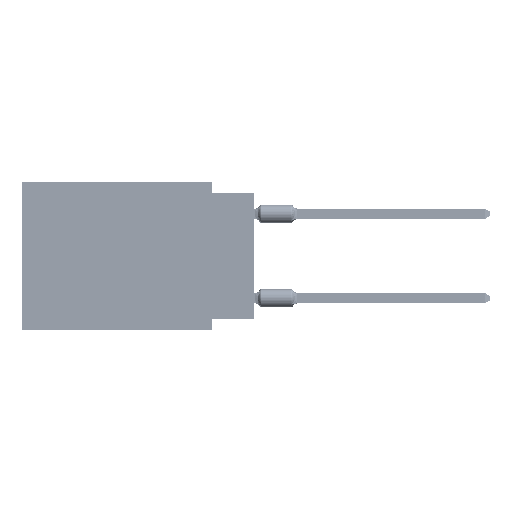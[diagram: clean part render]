
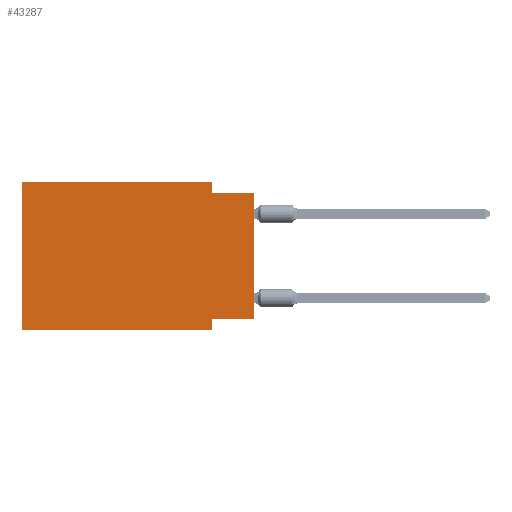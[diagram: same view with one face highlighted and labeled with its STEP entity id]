
A CAD part, left-side view. The second image highlights one B-rep face of the part: STEP entity #43287.
In plain terms, the highlighted planar face has unit normal (-1, 0, 0).
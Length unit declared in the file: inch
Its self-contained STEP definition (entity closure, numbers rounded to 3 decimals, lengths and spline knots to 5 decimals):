
#4055 = VECTOR ( 'NONE', #71321, 39.37008 ) ;
#4350 = VERTEX_POINT ( 'NONE', #39939 ) ;
#8627 = LINE ( 'NONE', #108207, #74319 ) ;
#8752 = VERTEX_POINT ( 'NONE', #32799 ) ;
#10209 = CARTESIAN_POINT ( 'NONE',  ( 0., 0., -0.025 ) ) ;
#11160 = DIRECTION ( 'NONE',  ( 0., 0., 1. ) ) ;
#11512 = CARTESIAN_POINT ( 'NONE',  ( 0., 0., -0.325 ) ) ;
#12114 = CARTESIAN_POINT ( 'NONE',  ( 0., 0.55, -0.35 ) ) ;
#12260 = ORIENTED_EDGE ( 'NONE', *, *, #32055, .T. ) ;
#14042 = VERTEX_POINT ( 'NONE', #77838 ) ;
#15272 = VECTOR ( 'NONE', #106214, 39.37008 ) ;
#15447 = EDGE_CURVE ( 'NONE', #56225, #14042, #8627, .T. ) ;
#16925 = DIRECTION ( 'NONE',  ( 0., 0., -1. ) ) ;
#19380 = ORIENTED_EDGE ( 'NONE', *, *, #62951, .F. ) ;
#21903 = VERTEX_POINT ( 'NONE', #11512 ) ;
#22581 = ORIENTED_EDGE ( 'NONE', *, *, #30645, .F. ) ;
#22696 = LINE ( 'NONE', #89085, #15272 ) ;
#24093 = CARTESIAN_POINT ( 'NONE',  ( 0., 0.1, -0.325 ) ) ;
#24596 = VECTOR ( 'NONE', #11160, 39.37008 ) ;
#25151 = CARTESIAN_POINT ( 'NONE',  ( 0., 0.55, 0. ) ) ;
#25230 = EDGE_CURVE ( 'NONE', #21903, #105555, #95223, .T. ) ;
#25435 = CARTESIAN_POINT ( 'NONE',  ( 0., 0., -0.325 ) ) ;
#25860 = DIRECTION ( 'NONE',  ( 0., -1., 0. ) ) ;
#29530 = CARTESIAN_POINT ( 'NONE',  ( 0., 0.55, 0. ) ) ;
#29986 = ORIENTED_EDGE ( 'NONE', *, *, #70982, .F. ) ;
#30645 = EDGE_CURVE ( 'NONE', #21903, #56225, #42617, .T. ) ;
#32055 = EDGE_CURVE ( 'NONE', #38311, #14042, #88986, .T. ) ;
#32799 = CARTESIAN_POINT ( 'NONE',  ( 0., 0.55, 0. ) ) ;
#32809 = AXIS2_PLACEMENT_3D ( 'NONE', #25151, #92608, #77106 ) ;
#34177 = LINE ( 'NONE', #67895, #62519 ) ;
#37190 = VECTOR ( 'NONE', #96983, 39.37008 ) ;
#38311 = VERTEX_POINT ( 'NONE', #40874 ) ;
#39939 = CARTESIAN_POINT ( 'NONE',  ( 0., 0.1, -0.025 ) ) ;
#40874 = CARTESIAN_POINT ( 'NONE',  ( 0., 0.55, -0.35 ) ) ;
#42617 = LINE ( 'NONE', #25435, #72996 ) ;
#43287 = ADVANCED_FACE ( 'NONE', ( #102017 ), #100930, .F. ) ;
#43338 = EDGE_LOOP ( 'NONE', ( #56687, #19380, #85348, #29986, #90044, #12260, #63796, #22581 ) ) ;
#49837 = EDGE_CURVE ( 'NONE', #90255, #4350, #76809, .T. ) ;
#56225 = VERTEX_POINT ( 'NONE', #24093 ) ;
#56687 = ORIENTED_EDGE ( 'NONE', *, *, #25230, .T. ) ;
#56701 = EDGE_CURVE ( 'NONE', #38311, #8752, #22696, .T. ) ;
#59151 = DIRECTION ( 'NONE',  ( 0., 0., -1. ) ) ;
#62519 = VECTOR ( 'NONE', #25860, 39.37008 ) ;
#62641 = CARTESIAN_POINT ( 'NONE',  ( 0., 0.1, 0. ) ) ;
#62951 = EDGE_CURVE ( 'NONE', #4350, #105555, #34177, .T. ) ;
#63796 = ORIENTED_EDGE ( 'NONE', *, *, #15447, .F. ) ;
#67895 = CARTESIAN_POINT ( 'NONE',  ( 0., 0., -0.025 ) ) ;
#70982 = EDGE_CURVE ( 'NONE', #8752, #90255, #105289, .T. ) ;
#71321 = DIRECTION ( 'NONE',  ( 0., -1., 0. ) ) ;
#72996 = VECTOR ( 'NONE', #94524, 39.37008 ) ;
#74319 = VECTOR ( 'NONE', #16925, 39.37008 ) ;
#76809 = LINE ( 'NONE', #85123, #91729 ) ;
#77106 = DIRECTION ( 'NONE',  ( 0., 0., -1. ) ) ;
#77838 = CARTESIAN_POINT ( 'NONE',  ( 0., 0.1, -0.35 ) ) ;
#85123 = CARTESIAN_POINT ( 'NONE',  ( 0., 0.1, 0. ) ) ;
#85348 = ORIENTED_EDGE ( 'NONE', *, *, #49837, .F. ) ;
#86948 = CARTESIAN_POINT ( 'NONE',  ( 0., 0., 0. ) ) ;
#88986 = LINE ( 'NONE', #12114, #4055 ) ;
#89085 = CARTESIAN_POINT ( 'NONE',  ( 0., 0.55, 0. ) ) ;
#90044 = ORIENTED_EDGE ( 'NONE', *, *, #56701, .F. ) ;
#90255 = VERTEX_POINT ( 'NONE', #62641 ) ;
#91729 = VECTOR ( 'NONE', #59151, 39.37008 ) ;
#92608 = DIRECTION ( 'NONE',  ( 1., 0., 0. ) ) ;
#94524 = DIRECTION ( 'NONE',  ( 0., 1., 0. ) ) ;
#95223 = LINE ( 'NONE', #86948, #24596 ) ;
#96983 = DIRECTION ( 'NONE',  ( 0., -1., 0. ) ) ;
#100930 = PLANE ( 'NONE',  #32809 ) ;
#102017 = FACE_OUTER_BOUND ( 'NONE', #43338, .T. ) ;
#105289 = LINE ( 'NONE', #29530, #37190 ) ;
#105555 = VERTEX_POINT ( 'NONE', #10209 ) ;
#106214 = DIRECTION ( 'NONE',  ( 0., 0., 1. ) ) ;
#108207 = CARTESIAN_POINT ( 'NONE',  ( 0., 0.1, -0.35 ) ) ;
